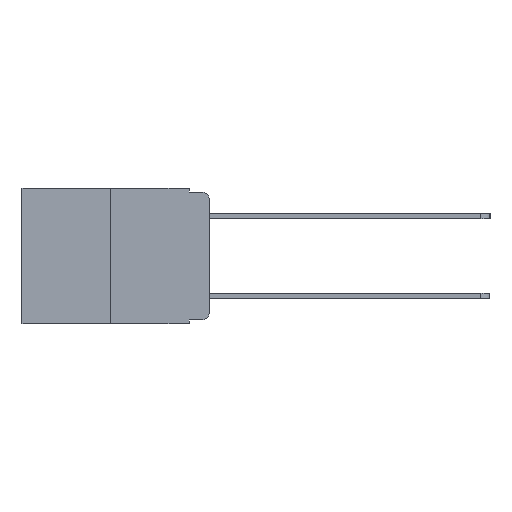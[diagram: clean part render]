
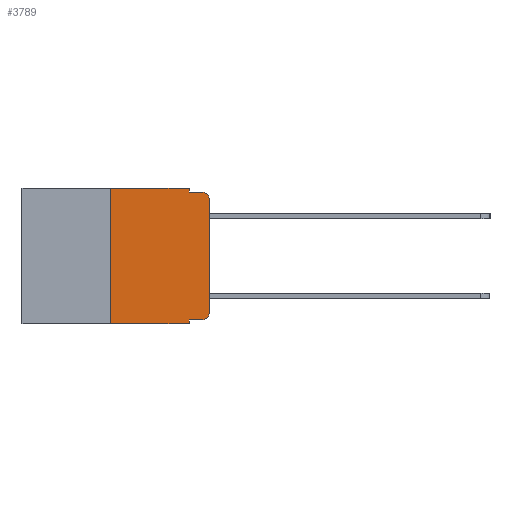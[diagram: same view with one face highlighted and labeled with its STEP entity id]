
A CAD part, left-side view. The second image highlights one B-rep face of the part: STEP entity #3789.
In plain terms, the highlighted planar face has unit normal (-1, 0, 0).
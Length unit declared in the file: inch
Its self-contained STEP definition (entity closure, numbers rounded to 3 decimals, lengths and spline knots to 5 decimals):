
#244 = VERTEX_POINT ( 'NONE', #13471 ) ;
#329 = CARTESIAN_POINT ( 'NONE',  ( 0., 0.051, -0.333 ) ) ;
#416 = CARTESIAN_POINT ( 'NONE',  ( 0., 0., -0.03 ) ) ;
#476 = EDGE_CURVE ( 'NONE', #9969, #2790, #14156, .T. ) ;
#515 = CARTESIAN_POINT ( 'NONE',  ( 0., 0.25, 0. ) ) ;
#729 = EDGE_CURVE ( 'NONE', #13241, #2722, #1394, .T. ) ;
#1156 = DIRECTION ( 'NONE',  ( 0., 0., -1. ) ) ;
#1205 = CARTESIAN_POINT ( 'NONE',  ( 0., 0.25, 0. ) ) ;
#1394 = LINE ( 'NONE', #11806, #12830 ) ;
#1652 = EDGE_CURVE ( 'NONE', #2421, #244, #2975, .T. ) ;
#1828 = CARTESIAN_POINT ( 'NONE',  ( 0., 0., -0.313 ) ) ;
#1940 = ORIENTED_EDGE ( 'NONE', *, *, #10670, .F. ) ;
#2421 = VERTEX_POINT ( 'NONE', #416 ) ;
#2543 = DIRECTION ( 'NONE',  ( 0., 0., 1. ) ) ;
#2722 = VERTEX_POINT ( 'NONE', #8890 ) ;
#2790 = VERTEX_POINT ( 'NONE', #10663 ) ;
#2950 = CARTESIAN_POINT ( 'NONE',  ( 0., 0.051, 0. ) ) ;
#2975 = CIRCLE ( 'NONE', #11098, 0.02 ) ;
#3011 = ORIENTED_EDGE ( 'NONE', *, *, #12816, .T. ) ;
#3110 = DIRECTION ( 'NONE',  ( 0., 0., -1. ) ) ;
#3257 = DIRECTION ( 'NONE',  ( -1., 0., 0. ) ) ;
#3528 = ORIENTED_EDGE ( 'NONE', *, *, #14066, .F. ) ;
#3789 = ADVANCED_FACE ( 'NONE', ( #12680 ), #10004, .F. ) ;
#3795 = VECTOR ( 'NONE', #8279, 39.37008 ) ;
#3938 = CARTESIAN_POINT ( 'NONE',  ( 0., 0.25, -0.343 ) ) ;
#3999 = LINE ( 'NONE', #9627, #9880 ) ;
#4078 = CARTESIAN_POINT ( 'NONE',  ( 0., 0., 0. ) ) ;
#4144 = ORIENTED_EDGE ( 'NONE', *, *, #1652, .T. ) ;
#4145 = ORIENTED_EDGE ( 'NONE', *, *, #6741, .T. ) ;
#4287 = CARTESIAN_POINT ( 'NONE',  ( 0., 0.473, 0. ) ) ;
#4377 = CARTESIAN_POINT ( 'NONE',  ( 0., 0.051, 0. ) ) ;
#4680 = ORIENTED_EDGE ( 'NONE', *, *, #729, .F. ) ;
#4988 = CARTESIAN_POINT ( 'NONE',  ( 0., 0.473, -0.343 ) ) ;
#4992 = VECTOR ( 'NONE', #6549, 39.37008 ) ;
#5180 = VECTOR ( 'NONE', #8508, 39.37008 ) ;
#5369 = ORIENTED_EDGE ( 'NONE', *, *, #14218, .F. ) ;
#5376 = VERTEX_POINT ( 'NONE', #11088 ) ;
#6243 = VECTOR ( 'NONE', #8258, 39.37008 ) ;
#6395 = CARTESIAN_POINT ( 'NONE',  ( 0., 0.051, -0.333 ) ) ;
#6511 = DIRECTION ( 'NONE',  ( 0., -1., 0. ) ) ;
#6549 = DIRECTION ( 'NONE',  ( 0., 0., 1. ) ) ;
#6669 = ORIENTED_EDGE ( 'NONE', *, *, #13770, .T. ) ;
#6741 = EDGE_CURVE ( 'NONE', #7586, #2421, #13753, .T. ) ;
#6952 = CARTESIAN_POINT ( 'NONE',  ( 0., 0.02, -0.313 ) ) ;
#7052 = LINE ( 'NONE', #4287, #12009 ) ;
#7586 = VERTEX_POINT ( 'NONE', #1828 ) ;
#7989 = DIRECTION ( 'NONE',  ( 0., 0., -1. ) ) ;
#8222 = VERTEX_POINT ( 'NONE', #3938 ) ;
#8258 = DIRECTION ( 'NONE',  ( 0., 0., -1. ) ) ;
#8279 = DIRECTION ( 'NONE',  ( 0., -1., 0. ) ) ;
#8508 = DIRECTION ( 'NONE',  ( 0., -1., 0. ) ) ;
#8890 = CARTESIAN_POINT ( 'NONE',  ( 0., 0.051, -0.01 ) ) ;
#8954 = AXIS2_PLACEMENT_3D ( 'NONE', #9981, #11659, #10537 ) ;
#9116 = LINE ( 'NONE', #1205, #13346 ) ;
#9627 = CARTESIAN_POINT ( 'NONE',  ( 0., 0.051, -0.01 ) ) ;
#9727 = LINE ( 'NONE', #4988, #3795 ) ;
#9880 = VECTOR ( 'NONE', #6511, 39.37008 ) ;
#9969 = VERTEX_POINT ( 'NONE', #329 ) ;
#9981 = CARTESIAN_POINT ( 'NONE',  ( 0., 0.473, 0. ) ) ;
#10004 = PLANE ( 'NONE',  #8954 ) ;
#10222 = VERTEX_POINT ( 'NONE', #515 ) ;
#10257 = ORIENTED_EDGE ( 'NONE', *, *, #476, .F. ) ;
#10366 = ORIENTED_EDGE ( 'NONE', *, *, #13442, .T. ) ;
#10537 = DIRECTION ( 'NONE',  ( 0., 0., -1. ) ) ;
#10663 = CARTESIAN_POINT ( 'NONE',  ( 0., 0.051, -0.343 ) ) ;
#10670 = EDGE_CURVE ( 'NONE', #10222, #13241, #7052, .T. ) ;
#10873 = LINE ( 'NONE', #6395, #5180 ) ;
#10945 = EDGE_LOOP ( 'NONE', ( #4145, #4144, #5369, #4680, #1940, #3528, #6669, #10257, #3011, #10366 ) ) ;
#11088 = CARTESIAN_POINT ( 'NONE',  ( 0., 0.02, -0.333 ) ) ;
#11098 = AXIS2_PLACEMENT_3D ( 'NONE', #13498, #3257, #3110 ) ;
#11659 = DIRECTION ( 'NONE',  ( 1., 0., 0. ) ) ;
#11806 = CARTESIAN_POINT ( 'NONE',  ( 0., 0.051, 0. ) ) ;
#12009 = VECTOR ( 'NONE', #13639, 39.37008 ) ;
#12473 = CIRCLE ( 'NONE', #12867, 0.02 ) ;
#12680 = FACE_OUTER_BOUND ( 'NONE', #10945, .T. ) ;
#12816 = EDGE_CURVE ( 'NONE', #9969, #5376, #10873, .T. ) ;
#12830 = VECTOR ( 'NONE', #1156, 39.37008 ) ;
#12867 = AXIS2_PLACEMENT_3D ( 'NONE', #6952, #13814, #7989 ) ;
#13241 = VERTEX_POINT ( 'NONE', #2950 ) ;
#13346 = VECTOR ( 'NONE', #2543, 39.37008 ) ;
#13442 = EDGE_CURVE ( 'NONE', #5376, #7586, #12473, .T. ) ;
#13471 = CARTESIAN_POINT ( 'NONE',  ( 0., 0.02, -0.01 ) ) ;
#13498 = CARTESIAN_POINT ( 'NONE',  ( 0., 0.02, -0.03 ) ) ;
#13639 = DIRECTION ( 'NONE',  ( 0., -1., 0. ) ) ;
#13753 = LINE ( 'NONE', #4078, #4992 ) ;
#13770 = EDGE_CURVE ( 'NONE', #8222, #2790, #9727, .T. ) ;
#13814 = DIRECTION ( 'NONE',  ( -1., 0., 0. ) ) ;
#14066 = EDGE_CURVE ( 'NONE', #8222, #10222, #9116, .T. ) ;
#14156 = LINE ( 'NONE', #4377, #6243 ) ;
#14218 = EDGE_CURVE ( 'NONE', #2722, #244, #3999, .T. ) ;
